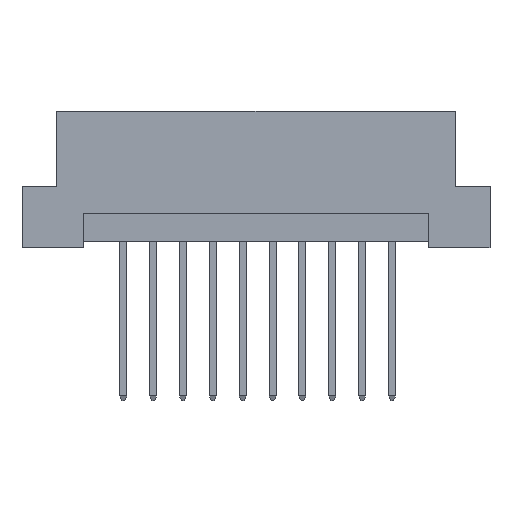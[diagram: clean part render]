
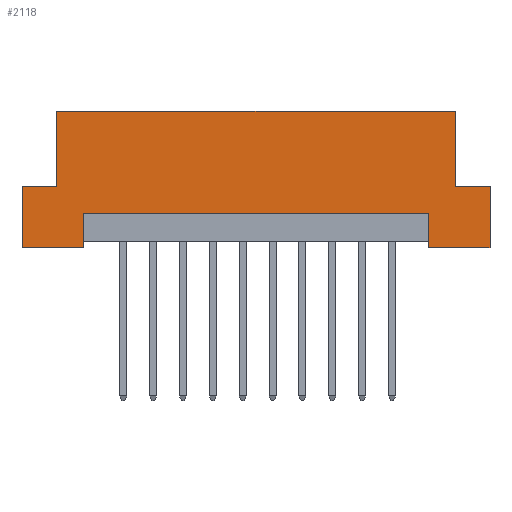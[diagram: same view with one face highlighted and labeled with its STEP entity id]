
A CAD part, front view. The second image highlights one B-rep face of the part: STEP entity #2118.
In plain terms, the highlighted planar face has unit normal (0, -1, 0).
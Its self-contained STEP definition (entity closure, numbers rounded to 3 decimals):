
#150 = CARTESIAN_POINT ( 'NONE',  ( 19.9, 0., 0. ) ) ;
#315 = CARTESIAN_POINT ( 'NONE',  ( 19.9, 0., 5.2 ) ) ;
#361 = ORIENTED_EDGE ( 'NONE', *, *, #6309, .F. ) ;
#547 = FACE_OUTER_BOUND ( 'NONE', #581, .T. ) ;
#572 = CARTESIAN_POINT ( 'NONE',  ( -19.9, 0., 0. ) ) ;
#581 = EDGE_LOOP ( 'NONE', ( #6743, #5582, #361, #1893, #985, #6119, #2317, #1135, #1659, #2557, #7076, #2592 ) ) ;
#673 = VERTEX_POINT ( 'NONE', #4270 ) ;
#826 = EDGE_CURVE ( 'NONE', #5964, #6182, #6892, .T. ) ;
#858 = CARTESIAN_POINT ( 'NONE',  ( -19.9, 0., 0. ) ) ;
#985 = ORIENTED_EDGE ( 'NONE', *, *, #1085, .F. ) ;
#1039 = CARTESIAN_POINT ( 'NONE',  ( -19.9, 0., 5.2 ) ) ;
#1043 = VECTOR ( 'NONE', #3508, 1000. ) ;
#1085 = EDGE_CURVE ( 'NONE', #6661, #7073, #5385, .T. ) ;
#1093 = EDGE_CURVE ( 'NONE', #6182, #3818, #4825, .T. ) ;
#1135 = ORIENTED_EDGE ( 'NONE', *, *, #7317, .F. ) ;
#1166 = DIRECTION ( 'NONE',  ( 0., 0., 1. ) ) ;
#1243 = PLANE ( 'NONE',  #2879 ) ;
#1269 = VERTEX_POINT ( 'NONE', #6846 ) ;
#1318 = VERTEX_POINT ( 'NONE', #2310 ) ;
#1324 = EDGE_CURVE ( 'NONE', #7073, #4291, #6988, .T. ) ;
#1390 = LINE ( 'NONE', #2493, #5855 ) ;
#1475 = VECTOR ( 'NONE', #5239, 1000. ) ;
#1483 = DIRECTION ( 'NONE',  ( 1., 0., 0. ) ) ;
#1585 = VECTOR ( 'NONE', #4401, 1000. ) ;
#1659 = ORIENTED_EDGE ( 'NONE', *, *, #1093, .F. ) ;
#1685 = LINE ( 'NONE', #572, #4301 ) ;
#1737 = VERTEX_POINT ( 'NONE', #3231 ) ;
#1820 = VECTOR ( 'NONE', #1483, 1000. ) ;
#1893 = ORIENTED_EDGE ( 'NONE', *, *, #1324, .F. ) ;
#1991 = DIRECTION ( 'NONE',  ( -1., 0., 0. ) ) ;
#2028 = CARTESIAN_POINT ( 'NONE',  ( -14.69, 0., 0.5 ) ) ;
#2118 = ADVANCED_FACE ( 'NONE', ( #547 ), #1243, .F. ) ;
#2140 = LINE ( 'NONE', #5498, #1585 ) ;
#2310 = CARTESIAN_POINT ( 'NONE',  ( 14.69, 0., 2.9 ) ) ;
#2317 = ORIENTED_EDGE ( 'NONE', *, *, #4547, .F. ) ;
#2359 = LINE ( 'NONE', #2432, #1475 ) ;
#2370 = EDGE_CURVE ( 'NONE', #1318, #7149, #2359, .T. ) ;
#2419 = DIRECTION ( 'NONE',  ( 0., 0., -1. ) ) ;
#2432 = CARTESIAN_POINT ( 'NONE',  ( 14.69, 0., 0.5 ) ) ;
#2464 = EDGE_CURVE ( 'NONE', #6661, #1737, #2140, .T. ) ;
#2493 = CARTESIAN_POINT ( 'NONE',  ( -16.94, 0., 5.2 ) ) ;
#2540 = LINE ( 'NONE', #2028, #7219 ) ;
#2557 = ORIENTED_EDGE ( 'NONE', *, *, #826, .F. ) ;
#2584 = DIRECTION ( 'NONE',  ( 1., 0., 0. ) ) ;
#2592 = ORIENTED_EDGE ( 'NONE', *, *, #5166, .F. ) ;
#2879 = AXIS2_PLACEMENT_3D ( 'NONE', #5052, #3366, #1166 ) ;
#2957 = CARTESIAN_POINT ( 'NONE',  ( -19.9, 0., 0. ) ) ;
#2985 = LINE ( 'NONE', #4145, #1043 ) ;
#3035 = CARTESIAN_POINT ( 'NONE',  ( 19.9, 0., 5.2 ) ) ;
#3082 = LINE ( 'NONE', #858, #6676 ) ;
#3118 = CARTESIAN_POINT ( 'NONE',  ( -14.69, 0., 0. ) ) ;
#3231 = CARTESIAN_POINT ( 'NONE',  ( 16.94, 0., 11.6 ) ) ;
#3334 = VECTOR ( 'NONE', #2419, 1000. ) ;
#3366 = DIRECTION ( 'NONE',  ( 0., 1., 0. ) ) ;
#3390 = DIRECTION ( 'NONE',  ( -1., 0., 0. ) ) ;
#3508 = DIRECTION ( 'NONE',  ( 1., 0., 0. ) ) ;
#3636 = DIRECTION ( 'NONE',  ( 0., 0., 1. ) ) ;
#3800 = CARTESIAN_POINT ( 'NONE',  ( 16.94, 0., 5.2 ) ) ;
#3818 = VERTEX_POINT ( 'NONE', #4314 ) ;
#4145 = CARTESIAN_POINT ( 'NONE',  ( -19.9, 0., 11.6 ) ) ;
#4225 = EDGE_CURVE ( 'NONE', #1318, #1269, #6555, .T. ) ;
#4270 = CARTESIAN_POINT ( 'NONE',  ( -16.94, 0., 11.6 ) ) ;
#4291 = VERTEX_POINT ( 'NONE', #6624 ) ;
#4301 = VECTOR ( 'NONE', #3390, 1000. ) ;
#4314 = CARTESIAN_POINT ( 'NONE',  ( -16.94, 0., 5.2 ) ) ;
#4401 = DIRECTION ( 'NONE',  ( 0., 0., 1. ) ) ;
#4547 = EDGE_CURVE ( 'NONE', #673, #1737, #2985, .T. ) ;
#4607 = VECTOR ( 'NONE', #6104, 1000. ) ;
#4709 = DIRECTION ( 'NONE',  ( 0., 0., 1. ) ) ;
#4825 = LINE ( 'NONE', #6588, #1820 ) ;
#5020 = VECTOR ( 'NONE', #2584, 1000. ) ;
#5052 = CARTESIAN_POINT ( 'NONE',  ( -19.9, 0., 11.6 ) ) ;
#5166 = EDGE_CURVE ( 'NONE', #1269, #7253, #2540, .T. ) ;
#5239 = DIRECTION ( 'NONE',  ( 0., 0., -1. ) ) ;
#5385 = LINE ( 'NONE', #315, #5020 ) ;
#5391 = CARTESIAN_POINT ( 'NONE',  ( 14.69, 0., 2.9 ) ) ;
#5491 = VECTOR ( 'NONE', #4709, 1000. ) ;
#5498 = CARTESIAN_POINT ( 'NONE',  ( 16.94, 0., 5.2 ) ) ;
#5582 = ORIENTED_EDGE ( 'NONE', *, *, #2370, .T. ) ;
#5855 = VECTOR ( 'NONE', #3636, 1000. ) ;
#5964 = VERTEX_POINT ( 'NONE', #2957 ) ;
#6104 = DIRECTION ( 'NONE',  ( -1., 0., 0. ) ) ;
#6119 = ORIENTED_EDGE ( 'NONE', *, *, #2464, .T. ) ;
#6144 = CARTESIAN_POINT ( 'NONE',  ( -19.9, 0., 0. ) ) ;
#6182 = VERTEX_POINT ( 'NONE', #1039 ) ;
#6309 = EDGE_CURVE ( 'NONE', #4291, #7149, #1685, .T. ) ;
#6535 = CARTESIAN_POINT ( 'NONE',  ( 14.69, 0., 0. ) ) ;
#6537 = DIRECTION ( 'NONE',  ( 0., 0., -1. ) ) ;
#6555 = LINE ( 'NONE', #5391, #4607 ) ;
#6588 = CARTESIAN_POINT ( 'NONE',  ( -19.9, 0., 5.2 ) ) ;
#6624 = CARTESIAN_POINT ( 'NONE',  ( 19.9, 0., 0. ) ) ;
#6661 = VERTEX_POINT ( 'NONE', #3800 ) ;
#6676 = VECTOR ( 'NONE', #1991, 1000. ) ;
#6723 = EDGE_CURVE ( 'NONE', #7253, #5964, #3082, .T. ) ;
#6743 = ORIENTED_EDGE ( 'NONE', *, *, #4225, .F. ) ;
#6846 = CARTESIAN_POINT ( 'NONE',  ( -14.69, 0., 2.9 ) ) ;
#6892 = LINE ( 'NONE', #6144, #5491 ) ;
#6988 = LINE ( 'NONE', #150, #3334 ) ;
#7073 = VERTEX_POINT ( 'NONE', #3035 ) ;
#7076 = ORIENTED_EDGE ( 'NONE', *, *, #6723, .F. ) ;
#7149 = VERTEX_POINT ( 'NONE', #6535 ) ;
#7219 = VECTOR ( 'NONE', #6537, 1000. ) ;
#7253 = VERTEX_POINT ( 'NONE', #3118 ) ;
#7317 = EDGE_CURVE ( 'NONE', #3818, #673, #1390, .T. ) ;
